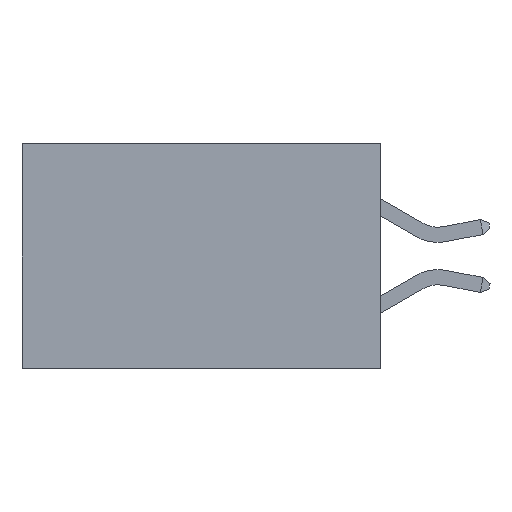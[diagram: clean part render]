
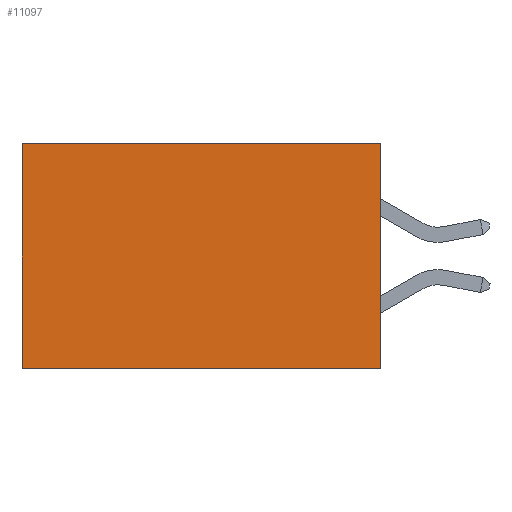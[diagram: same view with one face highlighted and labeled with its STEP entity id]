
A CAD part, left-side view. The second image highlights one B-rep face of the part: STEP entity #11097.
In plain terms, the highlighted planar face has unit normal (-1, 0, 0).
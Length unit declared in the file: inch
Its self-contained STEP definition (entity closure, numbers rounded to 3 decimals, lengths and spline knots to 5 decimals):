
#569 = ORIENTED_EDGE ( 'NONE', *, *, #28124, .F. ) ;
#2745 = VERTEX_POINT ( 'NONE', #25263 ) ;
#3049 = ORIENTED_EDGE ( 'NONE', *, *, #15583, .T. ) ;
#3539 = CARTESIAN_POINT ( 'NONE',  ( 0.277, 0.59, 0. ) ) ;
#5418 = VECTOR ( 'NONE', #25090, 39.37008 ) ;
#6859 = LINE ( 'NONE', #6979, #5418 ) ;
#6979 = CARTESIAN_POINT ( 'NONE',  ( 0.277, 0.59, -0.37 ) ) ;
#7853 = EDGE_CURVE ( 'NONE', #9081, #2745, #28457, .T. ) ;
#8210 = CARTESIAN_POINT ( 'NONE',  ( 0.277, 0., -0.37 ) ) ;
#8237 = DIRECTION ( 'NONE',  ( 0., 0., -1. ) ) ;
#8847 = CARTESIAN_POINT ( 'NONE',  ( 0.277, 0.59, -0.37 ) ) ;
#9081 = VERTEX_POINT ( 'NONE', #28610 ) ;
#9321 = DIRECTION ( 'NONE',  ( 1., 0., 0. ) ) ;
#9515 = DIRECTION ( 'NONE',  ( 0., 1., 0. ) ) ;
#10042 = VERTEX_POINT ( 'NONE', #8847 ) ;
#10540 = LINE ( 'NONE', #23126, #22634 ) ;
#11097 = ADVANCED_FACE ( 'NONE', ( #29236 ), #11539, .F. ) ;
#11539 = PLANE ( 'NONE',  #14123 ) ;
#14123 = AXIS2_PLACEMENT_3D ( 'NONE', #22939, #9321, #25146 ) ;
#14189 = LINE ( 'NONE', #25007, #26150 ) ;
#15583 = EDGE_CURVE ( 'NONE', #9081, #24922, #14189, .T. ) ;
#16090 = DIRECTION ( 'NONE',  ( 0., 1., 0. ) ) ;
#18971 = EDGE_LOOP ( 'NONE', ( #24252, #569, #23488, #3049 ) ) ;
#19361 = EDGE_CURVE ( 'NONE', #24922, #10042, #6859, .T. ) ;
#22634 = VECTOR ( 'NONE', #9515, 39.37008 ) ;
#22939 = CARTESIAN_POINT ( 'NONE',  ( 0.277, 0., -0.37 ) ) ;
#23126 = CARTESIAN_POINT ( 'NONE',  ( 0.277, 0., -0.37 ) ) ;
#23192 = VECTOR ( 'NONE', #8237, 39.37008 ) ;
#23488 = ORIENTED_EDGE ( 'NONE', *, *, #7853, .F. ) ;
#24252 = ORIENTED_EDGE ( 'NONE', *, *, #19361, .T. ) ;
#24922 = VERTEX_POINT ( 'NONE', #3539 ) ;
#25007 = CARTESIAN_POINT ( 'NONE',  ( 0.277, 0., 0. ) ) ;
#25090 = DIRECTION ( 'NONE',  ( 0., 0., -1. ) ) ;
#25146 = DIRECTION ( 'NONE',  ( 0., 0., -1. ) ) ;
#25263 = CARTESIAN_POINT ( 'NONE',  ( 0.277, 0., -0.37 ) ) ;
#26150 = VECTOR ( 'NONE', #16090, 39.37008 ) ;
#28124 = EDGE_CURVE ( 'NONE', #2745, #10042, #10540, .T. ) ;
#28457 = LINE ( 'NONE', #8210, #23192 ) ;
#28610 = CARTESIAN_POINT ( 'NONE',  ( 0.277, 0., 0. ) ) ;
#29236 = FACE_OUTER_BOUND ( 'NONE', #18971, .T. ) ;
